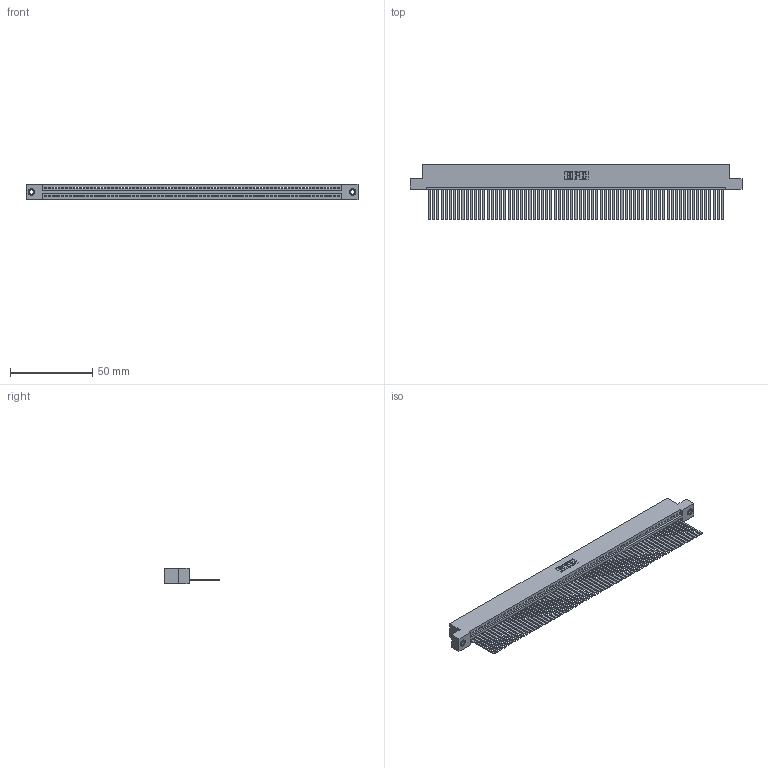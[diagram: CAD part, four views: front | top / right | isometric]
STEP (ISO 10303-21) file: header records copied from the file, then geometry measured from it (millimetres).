
FILE_DESCRIPTION (( 'STEP AP203' ), '1' );
FILE_NAME ('345-071-544-107.STEP', '2019-10-13T00:32:24', ( '' ), ( '' ), 'SwSTEP 2.0', 'SolidWorks 2016', '' );
FILE_SCHEMA (( 'CONFIG_CONTROL_DESIGN' ));
Length unit declared in the file: inch
Products named in the file (4): 345 Part_Flush Mounting Lugs - 0.156 Dia-TI; 345-071-544-107; 345-250-001_345-250-005-103; 345-292-001_345-293-144
Assembly tree (74 placements, depth 2):
  345-071-544-107
    345 Part_Flush Mounting Lugs - 0.156 Dia-TI
    345-292-001_345-293-144  x71
    345-250-001_345-250-005-103  x2
Bounding box: 201.55 x 33.96 x 9.4 mm (x, y, z)
Volume: 20189.6 mm3; surface area: 29725.5 mm2
Topology: 74 solids, 74 shells, 3878 faces, 11695 edges, 7694 vertices
Faces by surface type: plane 2668, cylinder 1194, cone 12, torus 4
Entity records: 50534 total; most frequent: CARTESIAN_POINT 8732, ORIENTED_EDGE 8730, DIRECTION 7609, EDGE_CURVE 4365, VECTOR 3933, LINE 3933, VERTEX_POINT 2904, AXIS2_PLACEMENT_3D 1838
